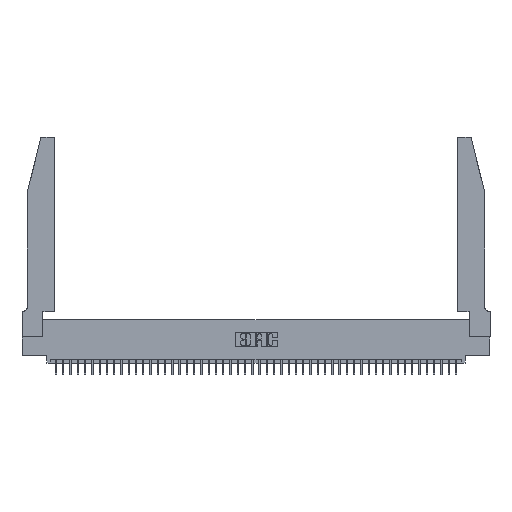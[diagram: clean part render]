
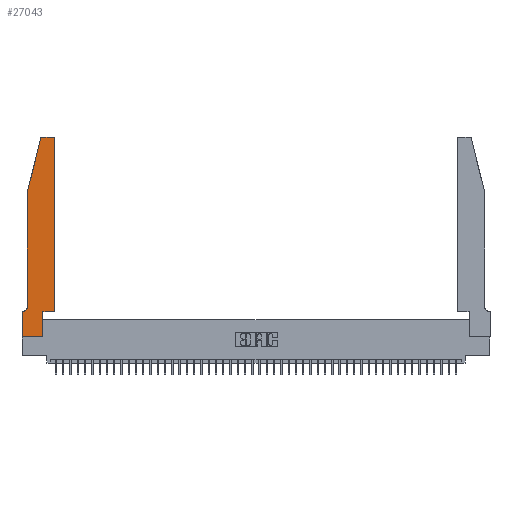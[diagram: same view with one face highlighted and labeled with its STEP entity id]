
A CAD part, top view. The second image highlights one B-rep face of the part: STEP entity #27043.
In plain terms, the highlighted planar face has unit normal (0, 0, 1).
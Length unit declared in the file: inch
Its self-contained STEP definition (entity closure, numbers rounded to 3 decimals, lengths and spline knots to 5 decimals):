
#1245 = CARTESIAN_POINT ( 'NONE',  ( 0., 0.35, 0.37 ) ) ;
#1639 = DIRECTION ( 'NONE',  ( 1., 0., 0. ) ) ;
#3140 = VERTEX_POINT ( 'NONE', #39133 ) ;
#3194 = CARTESIAN_POINT ( 'NONE',  ( 0.4205, 2.75, 0.37 ) ) ;
#4772 = CIRCLE ( 'NONE', #42311, 0.03 ) ;
#5117 = LINE ( 'NONE', #13281, #13709 ) ;
#5248 = VERTEX_POINT ( 'NONE', #25219 ) ;
#5474 = VECTOR ( 'NONE', #16905, 39.37008 ) ;
#5652 = VECTOR ( 'NONE', #42287, 39.37008 ) ;
#6383 = EDGE_CURVE ( 'NONE', #32659, #33212, #5117, .T. ) ;
#6605 = EDGE_CURVE ( 'NONE', #30184, #37548, #35267, .T. ) ;
#7775 = EDGE_CURVE ( 'NONE', #34203, #23607, #14223, .T. ) ;
#8009 = DIRECTION ( 'NONE',  ( 0., 0., 1. ) ) ;
#8636 = VERTEX_POINT ( 'NONE', #28314 ) ;
#8916 = LINE ( 'NONE', #34935, #5474 ) ;
#9100 = CARTESIAN_POINT ( 'NONE',  ( 0.2865, 0.35, 0.37 ) ) ;
#9163 = LINE ( 'NONE', #45420, #36943 ) ;
#9606 = EDGE_CURVE ( 'NONE', #35376, #26705, #8916, .T. ) ;
#9608 = ORIENTED_EDGE ( 'NONE', *, *, #16099, .T. ) ;
#10719 = EDGE_CURVE ( 'NONE', #8636, #32659, #26076, .T. ) ;
#11308 = ORIENTED_EDGE ( 'NONE', *, *, #7775, .T. ) ;
#13093 = CIRCLE ( 'NONE', #29880, 0.07 ) ;
#13102 = CARTESIAN_POINT ( 'NONE',  ( 0.4205, 2.72, 0.37 ) ) ;
#13130 = CARTESIAN_POINT ( 'NONE',  ( 0.0055, 0.42, 0.37 ) ) ;
#13281 = CARTESIAN_POINT ( 'NONE',  ( 0.2865, 0.35, 0.37 ) ) ;
#13709 = VECTOR ( 'NONE', #42240, 39.37008 ) ;
#13953 = EDGE_CURVE ( 'NONE', #26705, #30184, #4772, .T. ) ;
#14223 = LINE ( 'NONE', #38637, #5652 ) ;
#15499 = EDGE_LOOP ( 'NONE', ( #40739, #22631, #41882, #44138, #35660, #11308, #33978, #43605, #27760, #9608, #19240, #40784 ) ) ;
#16007 = VECTOR ( 'NONE', #32421, 39.37008 ) ;
#16099 = EDGE_CURVE ( 'NONE', #33212, #35376, #9163, .T. ) ;
#16730 = DIRECTION ( 'NONE',  ( 1., 0., 0. ) ) ;
#16767 = DIRECTION ( 'NONE',  ( -1., 0., 0. ) ) ;
#16905 = DIRECTION ( 'NONE',  ( 0., 1., 0. ) ) ;
#17956 = CARTESIAN_POINT ( 'NONE',  ( 0.0755, 2., 0.37 ) ) ;
#18383 = AXIS2_PLACEMENT_3D ( 'NONE', #29756, #8009, #33383 ) ;
#19240 = ORIENTED_EDGE ( 'NONE', *, *, #9606, .T. ) ;
#20169 = EDGE_CURVE ( 'NONE', #35706, #5248, #35816, .T. ) ;
#21169 = CARTESIAN_POINT ( 'NONE',  ( 0.284, 2.72, 0.37 ) ) ;
#21657 = CARTESIAN_POINT ( 'NONE',  ( 0.2605, 2.75, 0.37 ) ) ;
#21760 = LINE ( 'NONE', #43595, #24020 ) ;
#21929 = DIRECTION ( 'NONE',  ( 0., -1., 0. ) ) ;
#22027 = AXIS2_PLACEMENT_3D ( 'NONE', #21169, #46466, #24814 ) ;
#22631 = ORIENTED_EDGE ( 'NONE', *, *, #25587, .T. ) ;
#23607 = VERTEX_POINT ( 'NONE', #1245 ) ;
#23810 = DIRECTION ( 'NONE',  ( -0.239, -0.971, 0. ) ) ;
#24020 = VECTOR ( 'NONE', #21929, 39.37008 ) ;
#24648 = CARTESIAN_POINT ( 'NONE',  ( 0.4505, 0.35, 0.37 ) ) ;
#24814 = DIRECTION ( 'NONE',  ( 1., 0., 0. ) ) ;
#25219 = CARTESIAN_POINT ( 'NONE',  ( 0.0755, 2., 0.37 ) ) ;
#25587 = EDGE_CURVE ( 'NONE', #37548, #35706, #27645, .T. ) ;
#25968 = LINE ( 'NONE', #17956, #45199 ) ;
#26076 = LINE ( 'NONE', #30766, #34550 ) ;
#26705 = VERTEX_POINT ( 'NONE', #34966 ) ;
#27043 = ADVANCED_FACE ( 'NONE', ( #44485 ), #40346, .T. ) ;
#27645 = CIRCLE ( 'NONE', #22027, 0.03 ) ;
#27760 = ORIENTED_EDGE ( 'NONE', *, *, #6383, .T. ) ;
#28013 = EDGE_CURVE ( 'NONE', #23607, #8636, #21760, .T. ) ;
#28314 = CARTESIAN_POINT ( 'NONE',  ( 0., 0., 0.37 ) ) ;
#29756 = CARTESIAN_POINT ( 'NONE',  ( 0., 0.35, 0.37 ) ) ;
#29880 = AXIS2_PLACEMENT_3D ( 'NONE', #13130, #38462, #16767 ) ;
#30184 = VERTEX_POINT ( 'NONE', #3194 ) ;
#30766 = CARTESIAN_POINT ( 'NONE',  ( 0., 0., 0.37 ) ) ;
#30902 = EDGE_CURVE ( 'NONE', #5248, #3140, #25968, .T. ) ;
#31050 = DIRECTION ( 'NONE',  ( 1., 0., 0. ) ) ;
#32421 = DIRECTION ( 'NONE',  ( -1., 0., 0. ) ) ;
#32659 = VERTEX_POINT ( 'NONE', #41797 ) ;
#33212 = VERTEX_POINT ( 'NONE', #9100 ) ;
#33225 = CARTESIAN_POINT ( 'NONE',  ( 0.25487, 2.72718, 0.37 ) ) ;
#33383 = DIRECTION ( 'NONE',  ( 1., 0., 0. ) ) ;
#33978 = ORIENTED_EDGE ( 'NONE', *, *, #28013, .T. ) ;
#34021 = CARTESIAN_POINT ( 'NONE',  ( 0.0055, 0.35, 0.37 ) ) ;
#34203 = VERTEX_POINT ( 'NONE', #34021 ) ;
#34550 = VECTOR ( 'NONE', #1639, 39.37008 ) ;
#34935 = CARTESIAN_POINT ( 'NONE',  ( 0.4505, 0.35, 0.37 ) ) ;
#34966 = CARTESIAN_POINT ( 'NONE',  ( 0.4505, 2.72, 0.37 ) ) ;
#35267 = LINE ( 'NONE', #21657, #16007 ) ;
#35376 = VERTEX_POINT ( 'NONE', #24648 ) ;
#35660 = ORIENTED_EDGE ( 'NONE', *, *, #45258, .T. ) ;
#35706 = VERTEX_POINT ( 'NONE', #33225 ) ;
#35816 = LINE ( 'NONE', #45468, #46566 ) ;
#36943 = VECTOR ( 'NONE', #31050, 39.37008 ) ;
#37548 = VERTEX_POINT ( 'NONE', #46666 ) ;
#38420 = DIRECTION ( 'NONE',  ( 0., 0., 1. ) ) ;
#38462 = DIRECTION ( 'NONE',  ( 0., 0., -1. ) ) ;
#38637 = CARTESIAN_POINT ( 'NONE',  ( 0.0755, 0.35, 0.37 ) ) ;
#39133 = CARTESIAN_POINT ( 'NONE',  ( 0.0755, 0.42, 0.37 ) ) ;
#40346 = PLANE ( 'NONE',  #18383 ) ;
#40739 = ORIENTED_EDGE ( 'NONE', *, *, #6605, .T. ) ;
#40784 = ORIENTED_EDGE ( 'NONE', *, *, #13953, .T. ) ;
#41797 = CARTESIAN_POINT ( 'NONE',  ( 0.2865, 0., 0.37 ) ) ;
#41882 = ORIENTED_EDGE ( 'NONE', *, *, #20169, .T. ) ;
#42240 = DIRECTION ( 'NONE',  ( 0., 1., 0. ) ) ;
#42287 = DIRECTION ( 'NONE',  ( -1., 0., 0. ) ) ;
#42311 = AXIS2_PLACEMENT_3D ( 'NONE', #13102, #38420, #16730 ) ;
#43269 = DIRECTION ( 'NONE',  ( 0., -1., 0. ) ) ;
#43595 = CARTESIAN_POINT ( 'NONE',  ( 0., 0., 0.37 ) ) ;
#43605 = ORIENTED_EDGE ( 'NONE', *, *, #10719, .T. ) ;
#44138 = ORIENTED_EDGE ( 'NONE', *, *, #30902, .T. ) ;
#44485 = FACE_OUTER_BOUND ( 'NONE', #15499, .T. ) ;
#45199 = VECTOR ( 'NONE', #43269, 39.37008 ) ;
#45258 = EDGE_CURVE ( 'NONE', #3140, #34203, #13093, .T. ) ;
#45420 = CARTESIAN_POINT ( 'NONE',  ( 0.4505, 0.35, 0.37 ) ) ;
#45468 = CARTESIAN_POINT ( 'NONE',  ( 0.0755, 2., 0.37 ) ) ;
#46466 = DIRECTION ( 'NONE',  ( 0., 0., 1. ) ) ;
#46566 = VECTOR ( 'NONE', #23810, 39.37008 ) ;
#46666 = CARTESIAN_POINT ( 'NONE',  ( 0.284, 2.75, 0.37 ) ) ;
